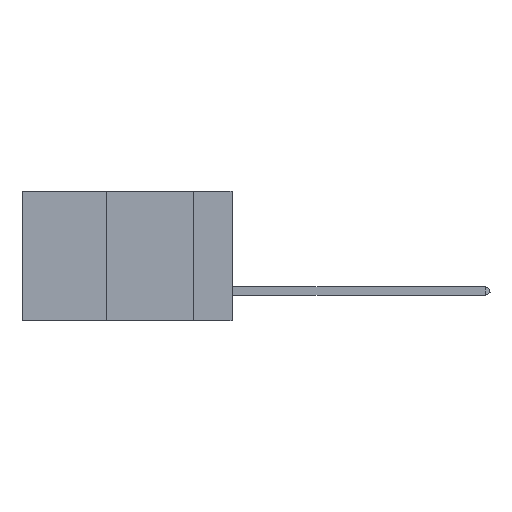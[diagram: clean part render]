
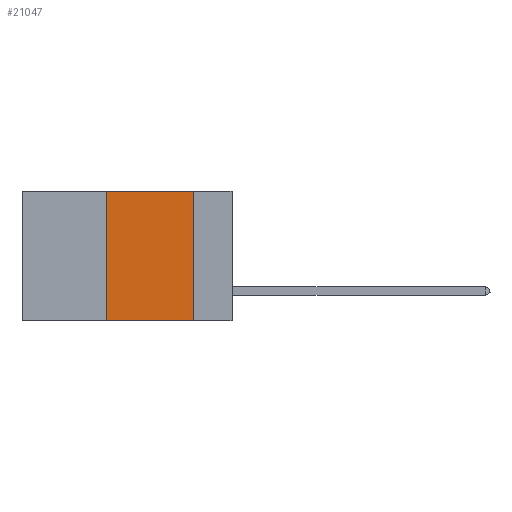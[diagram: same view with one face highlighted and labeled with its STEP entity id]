
A CAD part, left-side view. The second image highlights one B-rep face of the part: STEP entity #21047.
In plain terms, the highlighted planar face has unit normal (-1, 0, 0).
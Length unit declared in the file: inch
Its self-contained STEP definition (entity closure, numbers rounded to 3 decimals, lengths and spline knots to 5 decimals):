
#234 = AXIS2_PLACEMENT_3D ( 'NONE', #3102, #17232, #19195 ) ;
#1119 = CARTESIAN_POINT ( 'NONE',  ( 0., 0.6, -0.37 ) ) ;
#2460 = LINE ( 'NONE', #13072, #3412 ) ;
#3102 = CARTESIAN_POINT ( 'NONE',  ( 0., 0.6, 0. ) ) ;
#3412 = VECTOR ( 'NONE', #8688, 39.37008 ) ;
#4365 = LINE ( 'NONE', #16569, #14787 ) ;
#4438 = CARTESIAN_POINT ( 'NONE',  ( 0., 0.36, 0. ) ) ;
#4474 = VECTOR ( 'NONE', #23226, 39.37008 ) ;
#4539 = DIRECTION ( 'NONE',  ( 0., 0., -1. ) ) ;
#4555 = CARTESIAN_POINT ( 'NONE',  ( 0., 0.11, 0. ) ) ;
#4579 = ORIENTED_EDGE ( 'NONE', *, *, #20401, .T. ) ;
#4810 = LINE ( 'NONE', #4438, #24114 ) ;
#5576 = CARTESIAN_POINT ( 'NONE',  ( 0., 0.11, -0.37 ) ) ;
#5637 = VERTEX_POINT ( 'NONE', #10321 ) ;
#6147 = VERTEX_POINT ( 'NONE', #23714 ) ;
#7413 = ORIENTED_EDGE ( 'NONE', *, *, #8994, .F. ) ;
#8688 = DIRECTION ( 'NONE',  ( 0., -1., 0. ) ) ;
#8994 = EDGE_CURVE ( 'NONE', #22138, #14126, #4365, .T. ) ;
#9192 = LINE ( 'NONE', #1119, #4474 ) ;
#10126 = ORIENTED_EDGE ( 'NONE', *, *, #25845, .F. ) ;
#10321 = CARTESIAN_POINT ( 'NONE',  ( 0., 0.36, 0. ) ) ;
#12898 = FACE_OUTER_BOUND ( 'NONE', #19369, .T. ) ;
#13072 = CARTESIAN_POINT ( 'NONE',  ( 0., 0.6, 0. ) ) ;
#14126 = VERTEX_POINT ( 'NONE', #5576 ) ;
#14787 = VECTOR ( 'NONE', #4539, 39.37008 ) ;
#14935 = ORIENTED_EDGE ( 'NONE', *, *, #17580, .F. ) ;
#16569 = CARTESIAN_POINT ( 'NONE',  ( 0., 0.11, 0. ) ) ;
#17232 = DIRECTION ( 'NONE',  ( 1., 0., 0. ) ) ;
#17580 = EDGE_CURVE ( 'NONE', #6147, #5637, #4810, .T. ) ;
#19195 = DIRECTION ( 'NONE',  ( 0., 0., -1. ) ) ;
#19369 = EDGE_LOOP ( 'NONE', ( #7413, #10126, #14935, #4579 ) ) ;
#20401 = EDGE_CURVE ( 'NONE', #6147, #14126, #9192, .T. ) ;
#21047 = ADVANCED_FACE ( 'NONE', ( #12898 ), #21210, .F. ) ;
#21210 = PLANE ( 'NONE',  #234 ) ;
#22138 = VERTEX_POINT ( 'NONE', #4555 ) ;
#23068 = DIRECTION ( 'NONE',  ( 0., 0., 1. ) ) ;
#23226 = DIRECTION ( 'NONE',  ( 0., -1., 0. ) ) ;
#23714 = CARTESIAN_POINT ( 'NONE',  ( 0., 0.36, -0.37 ) ) ;
#24114 = VECTOR ( 'NONE', #23068, 39.37008 ) ;
#25845 = EDGE_CURVE ( 'NONE', #5637, #22138, #2460, .T. ) ;
